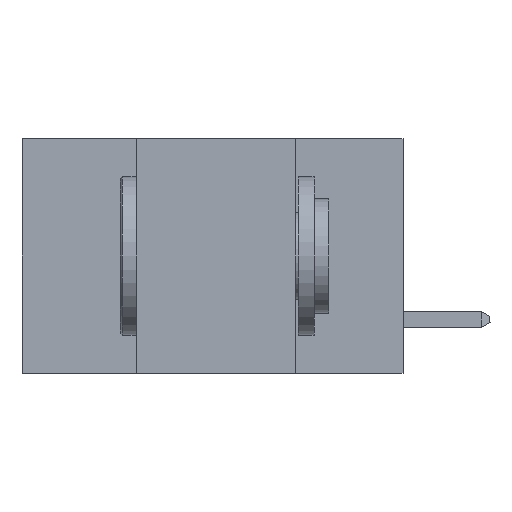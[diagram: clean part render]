
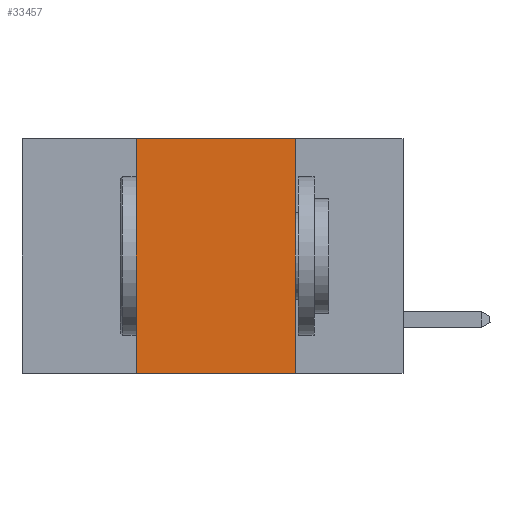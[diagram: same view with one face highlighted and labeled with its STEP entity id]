
A CAD part, left-side view. The second image highlights one B-rep face of the part: STEP entity #33457.
In plain terms, the highlighted planar face has unit normal (-1, 0, 0).
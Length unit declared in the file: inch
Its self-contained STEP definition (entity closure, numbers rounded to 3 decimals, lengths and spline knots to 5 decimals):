
#484 = VECTOR ( 'NONE', #41993, 39.37008 ) ;
#4046 = DIRECTION ( 'NONE',  ( 0., -1., 0. ) ) ;
#4534 = CARTESIAN_POINT ( 'NONE',  ( 0., 0.42, 0. ) ) ;
#4674 = VECTOR ( 'NONE', #24101, 39.37008 ) ;
#8420 = CARTESIAN_POINT ( 'NONE',  ( 0., 0.6, -0.37 ) ) ;
#12279 = CARTESIAN_POINT ( 'NONE',  ( 0., 0.17, -0.37 ) ) ;
#13028 = EDGE_CURVE ( 'NONE', #47158, #20558, #25052, .T. ) ;
#14884 = LINE ( 'NONE', #16530, #4674 ) ;
#14940 = LINE ( 'NONE', #23498, #484 ) ;
#16530 = CARTESIAN_POINT ( 'NONE',  ( 0., 0.42, 0. ) ) ;
#16612 = VECTOR ( 'NONE', #34901, 39.37008 ) ;
#17522 = CARTESIAN_POINT ( 'NONE',  ( 0., 0.42, -0.37 ) ) ;
#19506 = FACE_OUTER_BOUND ( 'NONE', #25132, .T. ) ;
#20558 = VERTEX_POINT ( 'NONE', #12279 ) ;
#21523 = ORIENTED_EDGE ( 'NONE', *, *, #13028, .T. ) ;
#21797 = ORIENTED_EDGE ( 'NONE', *, *, #44413, .F. ) ;
#23498 = CARTESIAN_POINT ( 'NONE',  ( 0., 0.17, 0. ) ) ;
#23560 = CARTESIAN_POINT ( 'NONE',  ( 0., 0.6, 0. ) ) ;
#24101 = DIRECTION ( 'NONE',  ( 0., 0., 1. ) ) ;
#25052 = LINE ( 'NONE', #8420, #16612 ) ;
#25132 = EDGE_LOOP ( 'NONE', ( #21797, #44573, #36056, #21523 ) ) ;
#26958 = DIRECTION ( 'NONE',  ( 0., 0., -1. ) ) ;
#30812 = DIRECTION ( 'NONE',  ( 1., 0., 0. ) ) ;
#32564 = VECTOR ( 'NONE', #4046, 39.37008 ) ;
#33457 = ADVANCED_FACE ( 'NONE', ( #19506 ), #46537, .F. ) ;
#34901 = DIRECTION ( 'NONE',  ( 0., -1., 0. ) ) ;
#36056 = ORIENTED_EDGE ( 'NONE', *, *, #37264, .F. ) ;
#37264 = EDGE_CURVE ( 'NONE', #47158, #39905, #14884, .T. ) ;
#39870 = EDGE_CURVE ( 'NONE', #39905, #42944, #46381, .T. ) ;
#39905 = VERTEX_POINT ( 'NONE', #4534 ) ;
#39970 = AXIS2_PLACEMENT_3D ( 'NONE', #23560, #30812, #26958 ) ;
#41656 = CARTESIAN_POINT ( 'NONE',  ( 0., 0.17, 0. ) ) ;
#41993 = DIRECTION ( 'NONE',  ( 0., 0., -1. ) ) ;
#42435 = CARTESIAN_POINT ( 'NONE',  ( 0., 0.6, 0. ) ) ;
#42944 = VERTEX_POINT ( 'NONE', #41656 ) ;
#44413 = EDGE_CURVE ( 'NONE', #42944, #20558, #14940, .T. ) ;
#44573 = ORIENTED_EDGE ( 'NONE', *, *, #39870, .F. ) ;
#46381 = LINE ( 'NONE', #42435, #32564 ) ;
#46537 = PLANE ( 'NONE',  #39970 ) ;
#47158 = VERTEX_POINT ( 'NONE', #17522 ) ;
